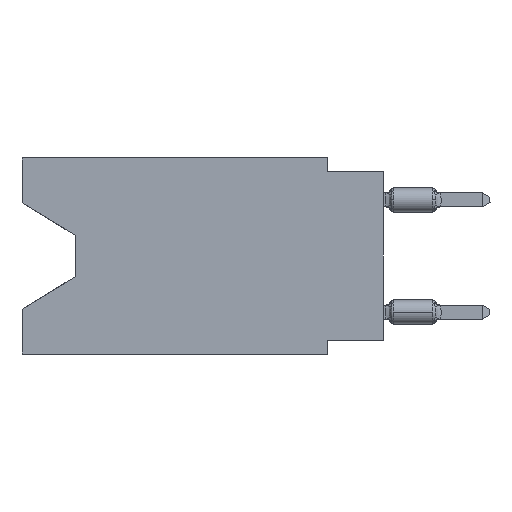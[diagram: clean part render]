
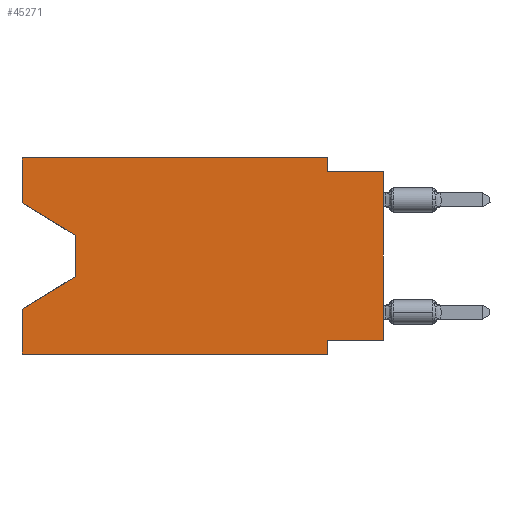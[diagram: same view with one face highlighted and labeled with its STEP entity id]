
A CAD part, left-side view. The second image highlights one B-rep face of the part: STEP entity #45271.
In plain terms, the highlighted planar face has unit normal (-1, 0, 0).
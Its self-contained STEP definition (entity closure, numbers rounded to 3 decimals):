
#430 = DIRECTION ( 'NONE',  ( 0., -1., 0. ) ) ;
#994 = ORIENTED_EDGE ( 'NONE', *, *, #19002, .F. ) ;
#1001 = CARTESIAN_POINT ( 'NONE',  ( 0., 2.54, 0. ) ) ;
#2002 = VECTOR ( 'NONE', #39764, 1000. ) ;
#2622 = ORIENTED_EDGE ( 'NONE', *, *, #38000, .F. ) ;
#3353 = VECTOR ( 'NONE', #9801, 1000. ) ;
#3774 = VERTEX_POINT ( 'NONE', #5581 ) ;
#4151 = VECTOR ( 'NONE', #24353, 1000. ) ;
#4184 = ORIENTED_EDGE ( 'NONE', *, *, #47024, .F. ) ;
#4355 = VECTOR ( 'NONE', #30627, 1000. ) ;
#4653 = ORIENTED_EDGE ( 'NONE', *, *, #23705, .T. ) ;
#4756 = DIRECTION ( 'NONE',  ( 0., 1., 0. ) ) ;
#5140 = DIRECTION ( 'NONE',  ( 0., 0., 1. ) ) ;
#5267 = AXIS2_PLACEMENT_3D ( 'NONE', #26132, #20186, #46412 ) ;
#5581 = CARTESIAN_POINT ( 'NONE',  ( 0., 16.383, 0. ) ) ;
#5793 = CARTESIAN_POINT ( 'NONE',  ( 0., 16.383, 0. ) ) ;
#6368 = ORIENTED_EDGE ( 'NONE', *, *, #20532, .T. ) ;
#6857 = EDGE_CURVE ( 'NONE', #51255, #62542, #47154, .T. ) ;
#7877 = CARTESIAN_POINT ( 'NONE',  ( 0., 16.383, -6.852 ) ) ;
#8217 = EDGE_CURVE ( 'NONE', #18879, #62542, #13130, .T. ) ;
#9039 = LINE ( 'NONE', #40315, #4151 ) ;
#9176 = CARTESIAN_POINT ( 'NONE',  ( 0., 0., -0.635 ) ) ;
#9801 = DIRECTION ( 'NONE',  ( 0., 0., 1. ) ) ;
#10301 = CARTESIAN_POINT ( 'NONE',  ( 0., 2.54, -8.89 ) ) ;
#10711 = VERTEX_POINT ( 'NONE', #7877 ) ;
#12912 = DIRECTION ( 'NONE',  ( 0., 0.855, -0.519 ) ) ;
#13130 = LINE ( 'NONE', #19467, #19014 ) ;
#13217 = CARTESIAN_POINT ( 'NONE',  ( 0., 13.97, -5.385 ) ) ;
#13746 = CARTESIAN_POINT ( 'NONE',  ( 0., 2.54, -8.255 ) ) ;
#15240 = CARTESIAN_POINT ( 'NONE',  ( 0., 16.383, -2.038 ) ) ;
#15667 = CARTESIAN_POINT ( 'NONE',  ( 0., 2.54, 0. ) ) ;
#18089 = VERTEX_POINT ( 'NONE', #15667 ) ;
#18861 = VECTOR ( 'NONE', #51214, 1000. ) ;
#18879 = VERTEX_POINT ( 'NONE', #25401 ) ;
#19002 = EDGE_CURVE ( 'NONE', #3774, #18089, #45350, .T. ) ;
#19014 = VECTOR ( 'NONE', #39741, 1000. ) ;
#19467 = CARTESIAN_POINT ( 'NONE',  ( 0., 16.383, -8.89 ) ) ;
#19542 = ORIENTED_EDGE ( 'NONE', *, *, #26845, .T. ) ;
#19616 = LINE ( 'NONE', #49210, #40343 ) ;
#20120 = CARTESIAN_POINT ( 'NONE',  ( 0., 13.97, -5.385 ) ) ;
#20186 = DIRECTION ( 'NONE',  ( 1., 0., 0. ) ) ;
#20532 = EDGE_CURVE ( 'NONE', #41869, #20884, #61358, .T. ) ;
#20884 = VERTEX_POINT ( 'NONE', #40620 ) ;
#20970 = ORIENTED_EDGE ( 'NONE', *, *, #8217, .T. ) ;
#22713 = LINE ( 'NONE', #42985, #28362 ) ;
#23381 = DIRECTION ( 'NONE',  ( 0., 0., -1. ) ) ;
#23705 = EDGE_CURVE ( 'NONE', #64535, #10711, #58477, .T. ) ;
#24353 = DIRECTION ( 'NONE',  ( 0., 0., 1. ) ) ;
#25401 = CARTESIAN_POINT ( 'NONE',  ( 0., 16.383, -8.89 ) ) ;
#25617 = EDGE_LOOP ( 'NONE', ( #6368, #19542, #4653, #48033, #20970, #33772, #65091, #63180, #35848, #4184, #994, #2622 ) ) ;
#26132 = CARTESIAN_POINT ( 'NONE',  ( 0., 16.383, 0. ) ) ;
#26794 = VERTEX_POINT ( 'NONE', #37371 ) ;
#26845 = EDGE_CURVE ( 'NONE', #20884, #64535, #22713, .T. ) ;
#28362 = VECTOR ( 'NONE', #23381, 1000. ) ;
#29601 = EDGE_CURVE ( 'NONE', #26794, #51255, #46314, .T. ) ;
#30627 = DIRECTION ( 'NONE',  ( 0., 0., -1. ) ) ;
#33772 = ORIENTED_EDGE ( 'NONE', *, *, #6857, .F. ) ;
#35287 = VECTOR ( 'NONE', #5140, 1000. ) ;
#35848 = ORIENTED_EDGE ( 'NONE', *, *, #45943, .F. ) ;
#35962 = VERTEX_POINT ( 'NONE', #9176 ) ;
#36071 = CARTESIAN_POINT ( 'NONE',  ( 0., 0., 0. ) ) ;
#36541 = CARTESIAN_POINT ( 'NONE',  ( 0., 2.54, -8.89 ) ) ;
#37371 = CARTESIAN_POINT ( 'NONE',  ( 0., 0., -8.255 ) ) ;
#38000 = EDGE_CURVE ( 'NONE', #41869, #3774, #9039, .T. ) ;
#39030 = VECTOR ( 'NONE', #430, 1000. ) ;
#39578 = DIRECTION ( 'NONE',  ( 0., -1., 0. ) ) ;
#39741 = DIRECTION ( 'NONE',  ( 0., -1., 0. ) ) ;
#39764 = DIRECTION ( 'NONE',  ( 0., -0.855, -0.519 ) ) ;
#40315 = CARTESIAN_POINT ( 'NONE',  ( 0., 16.383, 0. ) ) ;
#40343 = VECTOR ( 'NONE', #39578, 1000. ) ;
#40439 = CARTESIAN_POINT ( 'NONE',  ( 0., 16.383, -2.038 ) ) ;
#40620 = CARTESIAN_POINT ( 'NONE',  ( 0., 13.97, -3.505 ) ) ;
#40731 = LINE ( 'NONE', #5793, #3353 ) ;
#41869 = VERTEX_POINT ( 'NONE', #15240 ) ;
#42946 = CARTESIAN_POINT ( 'NONE',  ( 0., 2.54, -0.635 ) ) ;
#42985 = CARTESIAN_POINT ( 'NONE',  ( 0., 13.97, -3.505 ) ) ;
#44177 = VERTEX_POINT ( 'NONE', #42946 ) ;
#45271 = ADVANCED_FACE ( 'NONE', ( #51419 ), #65739, .F. ) ;
#45350 = LINE ( 'NONE', #61641, #39030 ) ;
#45943 = EDGE_CURVE ( 'NONE', #44177, #35962, #19616, .T. ) ;
#46256 = VECTOR ( 'NONE', #4756, 1000. ) ;
#46314 = LINE ( 'NONE', #60973, #46256 ) ;
#46412 = DIRECTION ( 'NONE',  ( 0., 0., -1. ) ) ;
#46565 = LINE ( 'NONE', #1001, #4355 ) ;
#47024 = EDGE_CURVE ( 'NONE', #18089, #44177, #46565, .T. ) ;
#47154 = LINE ( 'NONE', #36541, #18861 ) ;
#48033 = ORIENTED_EDGE ( 'NONE', *, *, #65695, .F. ) ;
#49210 = CARTESIAN_POINT ( 'NONE',  ( 0., 0., -0.635 ) ) ;
#51214 = DIRECTION ( 'NONE',  ( 0., 0., -1. ) ) ;
#51255 = VERTEX_POINT ( 'NONE', #13746 ) ;
#51419 = FACE_OUTER_BOUND ( 'NONE', #25617, .T. ) ;
#58477 = LINE ( 'NONE', #13217, #64847 ) ;
#60973 = CARTESIAN_POINT ( 'NONE',  ( 0., 0., -8.255 ) ) ;
#61358 = LINE ( 'NONE', #40439, #2002 ) ;
#61641 = CARTESIAN_POINT ( 'NONE',  ( 0., 16.383, 0. ) ) ;
#62542 = VERTEX_POINT ( 'NONE', #10301 ) ;
#63180 = ORIENTED_EDGE ( 'NONE', *, *, #65679, .T. ) ;
#64535 = VERTEX_POINT ( 'NONE', #20120 ) ;
#64847 = VECTOR ( 'NONE', #12912, 1000. ) ;
#65091 = ORIENTED_EDGE ( 'NONE', *, *, #29601, .F. ) ;
#65679 = EDGE_CURVE ( 'NONE', #26794, #35962, #65683, .T. ) ;
#65683 = LINE ( 'NONE', #36071, #35287 ) ;
#65695 = EDGE_CURVE ( 'NONE', #18879, #10711, #40731, .T. ) ;
#65739 = PLANE ( 'NONE',  #5267 ) ;
